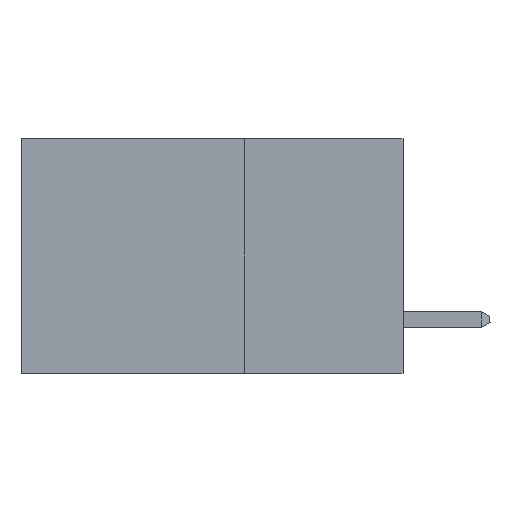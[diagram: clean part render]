
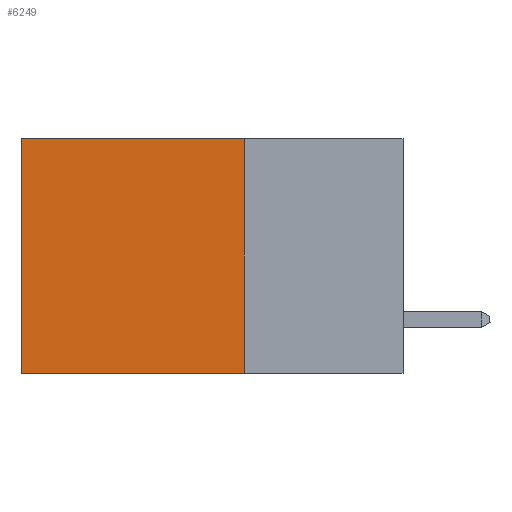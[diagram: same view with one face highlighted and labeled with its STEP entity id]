
A CAD part, left-side view. The second image highlights one B-rep face of the part: STEP entity #6249.
In plain terms, the highlighted planar face has unit normal (-1, 0, 0).
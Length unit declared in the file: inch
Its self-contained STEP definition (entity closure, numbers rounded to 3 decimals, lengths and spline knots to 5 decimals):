
#1247 = CARTESIAN_POINT ( 'NONE',  ( 0.2875, 0.6, 0. ) ) ;
#1364 = CARTESIAN_POINT ( 'NONE',  ( 0.2875, 0.6, 0. ) ) ;
#2723 = VERTEX_POINT ( 'NONE', #14885 ) ;
#3123 = VECTOR ( 'NONE', #18630, 39.37008 ) ;
#4378 = DIRECTION ( 'NONE',  ( 0., 1., 0. ) ) ;
#4430 = DIRECTION ( 'NONE',  ( 0., 1., 0. ) ) ;
#4963 = EDGE_LOOP ( 'NONE', ( #17928, #17995, #4981, #20311 ) ) ;
#4981 = ORIENTED_EDGE ( 'NONE', *, *, #6032, .F. ) ;
#5662 = VERTEX_POINT ( 'NONE', #1364 ) ;
#5916 = CARTESIAN_POINT ( 'NONE',  ( 0.2875, 0.25, -0.37 ) ) ;
#6032 = EDGE_CURVE ( 'NONE', #9278, #18671, #14470, .T. ) ;
#6035 = DIRECTION ( 'NONE',  ( 0., 0., -1. ) ) ;
#6072 = VECTOR ( 'NONE', #4430, 39.37008 ) ;
#6249 = ADVANCED_FACE ( 'NONE', ( #11576 ), #11435, .F. ) ;
#7683 = VECTOR ( 'NONE', #7756, 39.37008 ) ;
#7756 = DIRECTION ( 'NONE',  ( 0., 0., -1. ) ) ;
#7940 = CARTESIAN_POINT ( 'NONE',  ( 0.2875, 0.25, -0.37 ) ) ;
#9278 = VERTEX_POINT ( 'NONE', #21399 ) ;
#9330 = LINE ( 'NONE', #5916, #12497 ) ;
#9876 = EDGE_CURVE ( 'NONE', #18671, #2723, #9330, .T. ) ;
#11418 = EDGE_CURVE ( 'NONE', #9278, #5662, #14537, .T. ) ;
#11435 = PLANE ( 'NONE',  #12408 ) ;
#11444 = EDGE_CURVE ( 'NONE', #5662, #2723, #21618, .T. ) ;
#11576 = FACE_OUTER_BOUND ( 'NONE', #4963, .T. ) ;
#12408 = AXIS2_PLACEMENT_3D ( 'NONE', #16176, #14464, #6035 ) ;
#12497 = VECTOR ( 'NONE', #4378, 39.37008 ) ;
#14464 = DIRECTION ( 'NONE',  ( 1., 0., 0. ) ) ;
#14470 = LINE ( 'NONE', #16841, #3123 ) ;
#14537 = LINE ( 'NONE', #16106, #6072 ) ;
#14885 = CARTESIAN_POINT ( 'NONE',  ( 0.2875, 0.6, -0.37 ) ) ;
#16106 = CARTESIAN_POINT ( 'NONE',  ( 0.2875, 0.25, 0. ) ) ;
#16176 = CARTESIAN_POINT ( 'NONE',  ( 0.2875, 0.25, 0. ) ) ;
#16841 = CARTESIAN_POINT ( 'NONE',  ( 0.2875, 0.25, 0. ) ) ;
#17928 = ORIENTED_EDGE ( 'NONE', *, *, #11444, .T. ) ;
#17995 = ORIENTED_EDGE ( 'NONE', *, *, #9876, .F. ) ;
#18630 = DIRECTION ( 'NONE',  ( 0., 0., -1. ) ) ;
#18671 = VERTEX_POINT ( 'NONE', #7940 ) ;
#20311 = ORIENTED_EDGE ( 'NONE', *, *, #11418, .T. ) ;
#21399 = CARTESIAN_POINT ( 'NONE',  ( 0.2875, 0.25, 0. ) ) ;
#21618 = LINE ( 'NONE', #1247, #7683 ) ;
